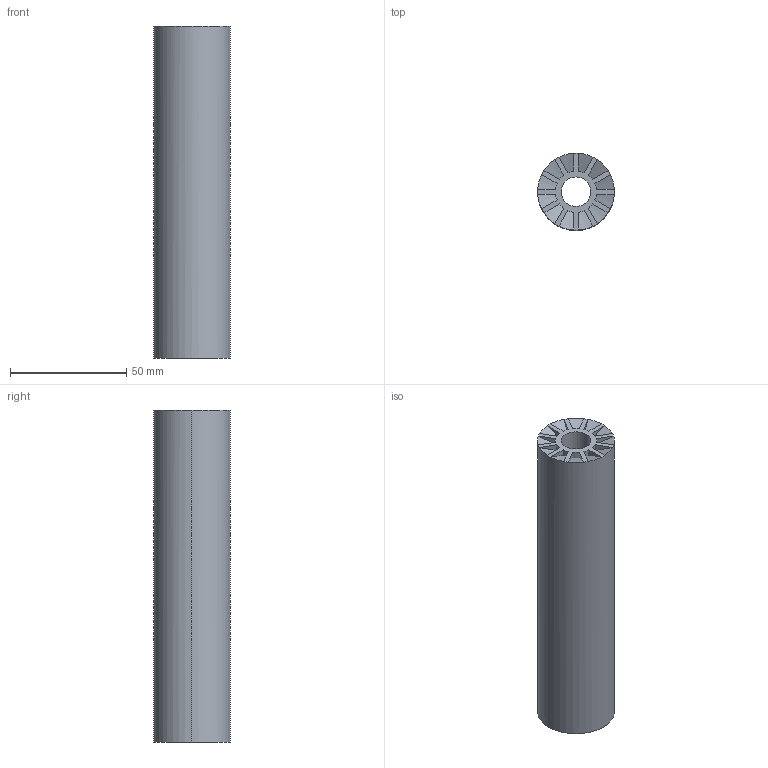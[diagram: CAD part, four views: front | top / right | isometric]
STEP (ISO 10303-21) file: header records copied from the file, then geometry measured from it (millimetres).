
FILE_DESCRIPTION (( 'STEP AP214' ), '1' );
FILE_NAME ('FauxCan.step', '2019-12-18T03:07:40', ( '' ), ( '' ), 'SwSTEP 2.0', 'SolidWorks 2019', '' );
FILE_SCHEMA (( 'AUTOMOTIVE_DESIGN' ));
Length unit declared in the file: millimetre
Products named in the file (1): FauxCan
Bounding box: 33 x 33 x 142.5 mm (x, y, z)
Volume: 45827.6 mm3; surface area: 29091.2 mm2
Topology: 1 solids, 1 shells, 111 faces, 256 edges, 148 vertices
Faces by surface type: plane 75, cylinder 20, cone 16
Entity records: 3100 total; most frequent: CARTESIAN_POINT 660, ORIENTED_EDGE 512, DIRECTION 484, EDGE_CURVE 256, AXIS2_PLACEMENT_3D 164, LINE 156, VECTOR 156, VERTEX_POINT 148
